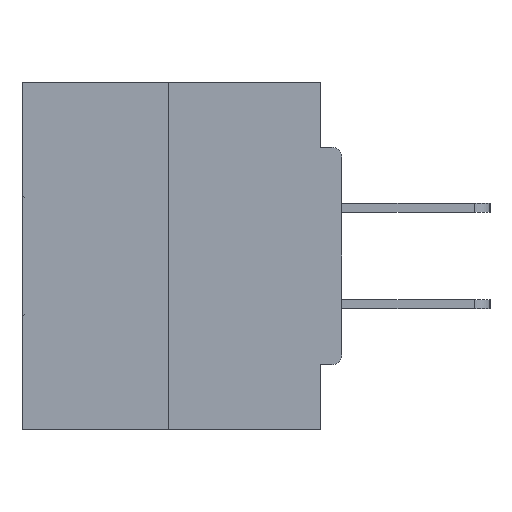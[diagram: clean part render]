
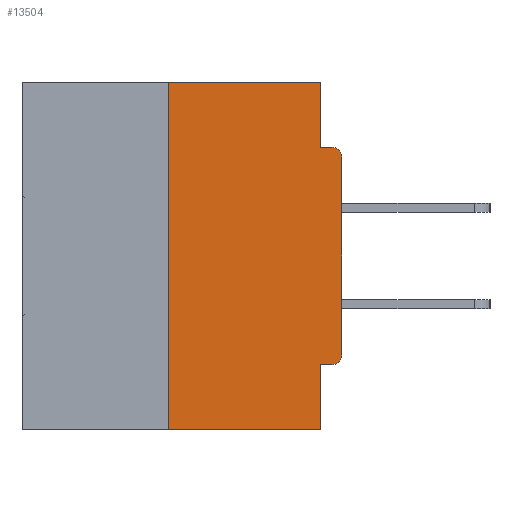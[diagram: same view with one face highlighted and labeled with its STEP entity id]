
A CAD part, left-side view. The second image highlights one B-rep face of the part: STEP entity #13504.
In plain terms, the highlighted planar face has unit normal (-1, 0, 0).
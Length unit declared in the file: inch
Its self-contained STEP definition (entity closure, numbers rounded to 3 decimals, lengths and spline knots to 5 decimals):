
#927 = EDGE_CURVE ( 'NONE', #20884, #16452, #30604, .T. ) ;
#1719 = VECTOR ( 'NONE', #1907, 39.37008 ) ;
#1907 = DIRECTION ( 'NONE',  ( 0., -1., 0. ) ) ;
#2187 = VERTEX_POINT ( 'NONE', #39296 ) ;
#2631 = VERTEX_POINT ( 'NONE', #27539 ) ;
#2770 = EDGE_CURVE ( 'NONE', #8973, #2631, #33500, .T. ) ;
#4550 = VECTOR ( 'NONE', #6533, 39.37008 ) ;
#4576 = VERTEX_POINT ( 'NONE', #12996 ) ;
#4759 = ORIENTED_EDGE ( 'NONE', *, *, #34442, .F. ) ;
#5735 = DIRECTION ( 'NONE',  ( 0., 0., 1. ) ) ;
#6279 = ORIENTED_EDGE ( 'NONE', *, *, #24703, .T. ) ;
#6374 = VECTOR ( 'NONE', #13964, 39.37008 ) ;
#6533 = DIRECTION ( 'NONE',  ( 0., 0., 1. ) ) ;
#7255 = EDGE_LOOP ( 'NONE', ( #4759, #34839, #41860, #34870, #8664, #16557, #30097, #6279, #14536, #25863 ) ) ;
#7385 = DIRECTION ( 'NONE',  ( 0., 0., -1. ) ) ;
#7931 = LINE ( 'NONE', #27123, #11006 ) ;
#8249 = VECTOR ( 'NONE', #5735, 39.37008 ) ;
#8664 = ORIENTED_EDGE ( 'NONE', *, *, #15339, .F. ) ;
#8973 = VERTEX_POINT ( 'NONE', #18578 ) ;
#10651 = CARTESIAN_POINT ( 'NONE',  ( 0., 0.031, -0.5 ) ) ;
#10717 = CARTESIAN_POINT ( 'NONE',  ( 0., 0.031, 0. ) ) ;
#10779 = CARTESIAN_POINT ( 'NONE',  ( 0., 0.46, 0. ) ) ;
#10944 = CARTESIAN_POINT ( 'NONE',  ( 0., 0.031, 0. ) ) ;
#11006 = VECTOR ( 'NONE', #14701, 39.37008 ) ;
#11027 = LINE ( 'NONE', #31733, #1719 ) ;
#11613 = VERTEX_POINT ( 'NONE', #19657 ) ;
#12010 = VECTOR ( 'NONE', #24461, 39.37008 ) ;
#12438 = CARTESIAN_POINT ( 'NONE',  ( 0., 0., -0.4065 ) ) ;
#12632 = EDGE_CURVE ( 'NONE', #4576, #11613, #22395, .T. ) ;
#12856 = CARTESIAN_POINT ( 'NONE',  ( 0., 0., 0. ) ) ;
#12996 = CARTESIAN_POINT ( 'NONE',  ( 0., 0.015, -0.4065 ) ) ;
#13504 = ADVANCED_FACE ( 'NONE', ( #38258 ), #24239, .F. ) ;
#13964 = DIRECTION ( 'NONE',  ( 0., 0., -1. ) ) ;
#14265 = VECTOR ( 'NONE', #40628, 39.37008 ) ;
#14536 = ORIENTED_EDGE ( 'NONE', *, *, #36992, .F. ) ;
#14701 = DIRECTION ( 'NONE',  ( 0., -1., 0. ) ) ;
#15339 = EDGE_CURVE ( 'NONE', #4576, #2187, #22118, .T. ) ;
#16452 = VERTEX_POINT ( 'NONE', #34806 ) ;
#16557 = ORIENTED_EDGE ( 'NONE', *, *, #12632, .T. ) ;
#16911 = CARTESIAN_POINT ( 'NONE',  ( 0., 0.015, -0.3915 ) ) ;
#17567 = CIRCLE ( 'NONE', #35671, 0.015 ) ;
#17632 = EDGE_CURVE ( 'NONE', #8973, #36635, #40062, .T. ) ;
#17745 = DIRECTION ( 'NONE',  ( 0., 0., -1. ) ) ;
#17801 = VERTEX_POINT ( 'NONE', #30237 ) ;
#18578 = CARTESIAN_POINT ( 'NONE',  ( 0., 0.25, -0.5 ) ) ;
#19446 = DIRECTION ( 'NONE',  ( 0., 0., -1. ) ) ;
#19657 = CARTESIAN_POINT ( 'NONE',  ( 0., 0., -0.3915 ) ) ;
#19725 = DIRECTION ( 'NONE',  ( -1., 0., 0. ) ) ;
#20884 = VERTEX_POINT ( 'NONE', #10944 ) ;
#22118 = LINE ( 'NONE', #12438, #39060 ) ;
#22236 = CARTESIAN_POINT ( 'NONE',  ( 0., 0.031, -0.5 ) ) ;
#22395 = CIRCLE ( 'NONE', #25036, 0.015 ) ;
#22637 = EDGE_CURVE ( 'NONE', #11613, #28118, #33420, .T. ) ;
#24239 = PLANE ( 'NONE',  #29722 ) ;
#24461 = DIRECTION ( 'NONE',  ( 0., 0., -1. ) ) ;
#24703 = EDGE_CURVE ( 'NONE', #28118, #17801, #17567, .T. ) ;
#25036 = AXIS2_PLACEMENT_3D ( 'NONE', #16911, #36922, #7385 ) ;
#25458 = LINE ( 'NONE', #10651, #6374 ) ;
#25863 = ORIENTED_EDGE ( 'NONE', *, *, #927, .F. ) ;
#27123 = CARTESIAN_POINT ( 'NONE',  ( 0., 0., -0.0935 ) ) ;
#27539 = CARTESIAN_POINT ( 'NONE',  ( 0., 0.25, 0. ) ) ;
#27669 = DIRECTION ( 'NONE',  ( 1., 0., 0. ) ) ;
#28118 = VERTEX_POINT ( 'NONE', #35994 ) ;
#29722 = AXIS2_PLACEMENT_3D ( 'NONE', #10779, #27669, #17745 ) ;
#30097 = ORIENTED_EDGE ( 'NONE', *, *, #22637, .T. ) ;
#30237 = CARTESIAN_POINT ( 'NONE',  ( 0., 0.015, -0.0935 ) ) ;
#30604 = LINE ( 'NONE', #10717, #12010 ) ;
#31684 = CARTESIAN_POINT ( 'NONE',  ( 0., 0.25, 0. ) ) ;
#31733 = CARTESIAN_POINT ( 'NONE',  ( 0., 0.46, 0. ) ) ;
#33420 = LINE ( 'NONE', #12856, #4550 ) ;
#33500 = LINE ( 'NONE', #31684, #8249 ) ;
#34442 = EDGE_CURVE ( 'NONE', #2631, #20884, #11027, .T. ) ;
#34806 = CARTESIAN_POINT ( 'NONE',  ( 0., 0.031, -0.0935 ) ) ;
#34839 = ORIENTED_EDGE ( 'NONE', *, *, #2770, .F. ) ;
#34870 = ORIENTED_EDGE ( 'NONE', *, *, #36973, .F. ) ;
#35275 = CARTESIAN_POINT ( 'NONE',  ( 0., 0.015, -0.1085 ) ) ;
#35671 = AXIS2_PLACEMENT_3D ( 'NONE', #35275, #19725, #19446 ) ;
#35994 = CARTESIAN_POINT ( 'NONE',  ( 0., 0., -0.1085 ) ) ;
#36635 = VERTEX_POINT ( 'NONE', #22236 ) ;
#36922 = DIRECTION ( 'NONE',  ( -1., 0., 0. ) ) ;
#36973 = EDGE_CURVE ( 'NONE', #2187, #36635, #25458, .T. ) ;
#36992 = EDGE_CURVE ( 'NONE', #16452, #17801, #7931, .T. ) ;
#37360 = CARTESIAN_POINT ( 'NONE',  ( 0., 0.46, -0.5 ) ) ;
#38258 = FACE_OUTER_BOUND ( 'NONE', #7255, .T. ) ;
#38658 = DIRECTION ( 'NONE',  ( 0., 1., 0. ) ) ;
#39060 = VECTOR ( 'NONE', #38658, 39.37008 ) ;
#39296 = CARTESIAN_POINT ( 'NONE',  ( 0., 0.031, -0.4065 ) ) ;
#40062 = LINE ( 'NONE', #37360, #14265 ) ;
#40628 = DIRECTION ( 'NONE',  ( 0., -1., 0. ) ) ;
#41860 = ORIENTED_EDGE ( 'NONE', *, *, #17632, .T. ) ;
